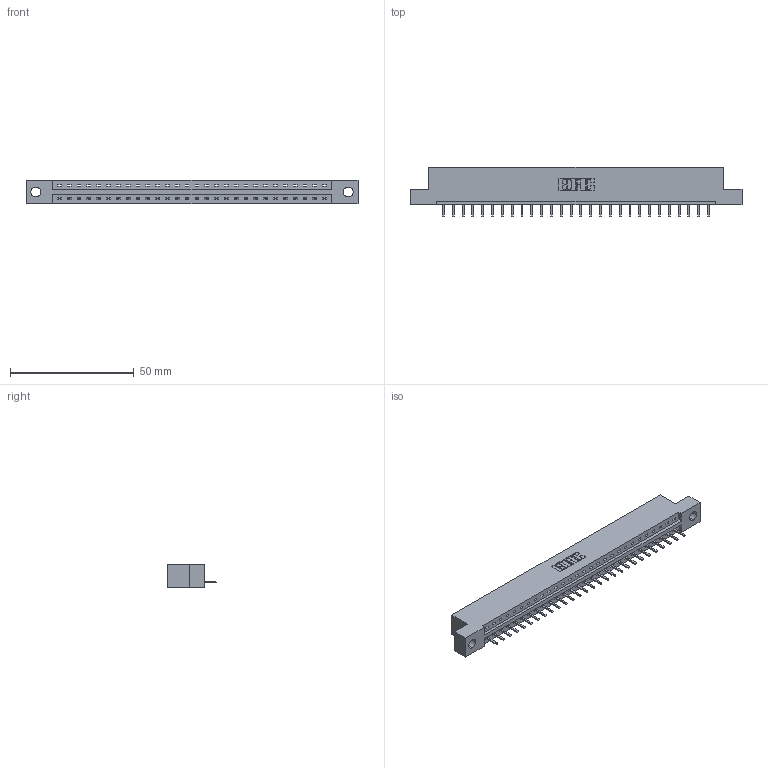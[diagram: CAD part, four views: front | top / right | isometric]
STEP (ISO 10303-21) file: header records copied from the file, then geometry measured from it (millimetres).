
FILE_DESCRIPTION (( 'STEP AP203' ), '1' );
FILE_NAME ('387-028-520-104.STEP', '2019-10-03T14:29:46', ( '' ), ( '' ), 'SwSTEP 2.0', 'SolidWorks 2016', '' );
FILE_SCHEMA (( 'CONFIG_CONTROL_DESIGN' ));
Length unit declared in the file: inch
Products named in the file (3): 337 Part_Flush Mounting Lugs - 0.156 Dia-TH; 345-292-001_345-293-120; 387-028-520-104
Assembly tree (29 placements, depth 2):
  387-028-520-104
    337 Part_Flush Mounting Lugs - 0.156 Dia-TH
    345-292-001_345-293-120  x28
Bounding box: 133.96 x 20.02 x 9.4 mm (x, y, z)
Volume: 13579.3 mm3; surface area: 13459.8 mm2
Topology: 29 solids, 29 shells, 1962 faces, 5799 edges, 3790 vertices
Faces by surface type: plane 1414, cylinder 548
Entity records: 22741 total; most frequent: CARTESIAN_POINT 3978, ORIENTED_EDGE 3930, DIRECTION 3365, EDGE_CURVE 1965, VECTOR 1833, LINE 1833, VERTEX_POINT 1306, AXIS2_PLACEMENT_3D 766
